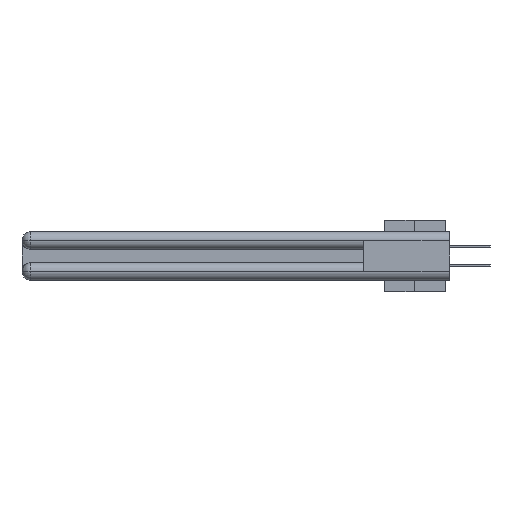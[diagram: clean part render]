
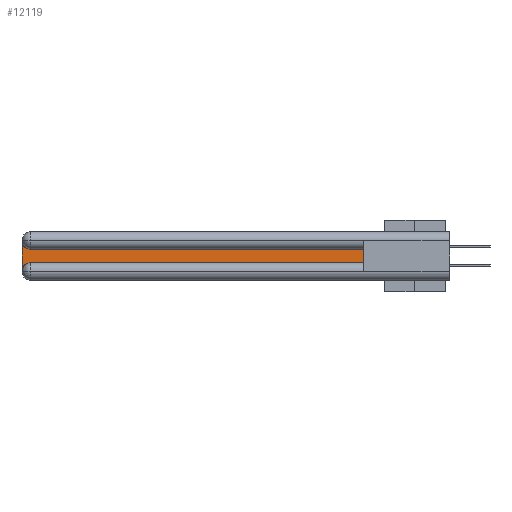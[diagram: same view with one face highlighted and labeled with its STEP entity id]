
A CAD part, left-side view. The second image highlights one B-rep face of the part: STEP entity #12119.
In plain terms, the highlighted planar face has unit normal (-1, 0, 0).
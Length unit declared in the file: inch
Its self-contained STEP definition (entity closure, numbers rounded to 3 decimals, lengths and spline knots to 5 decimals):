
#424 = AXIS2_PLACEMENT_3D ( 'NONE', #31968, #34974, #2307 ) ;
#792 = EDGE_CURVE ( 'NONE', #24513, #30034, #34742, .T. ) ;
#1741 = ORIENTED_EDGE ( 'NONE', *, *, #31828, .T. ) ;
#2096 = CIRCLE ( 'NONE', #424, 0.06 ) ;
#2307 = DIRECTION ( 'NONE',  ( 0., 0., -1. ) ) ;
#2764 = DIRECTION ( 'NONE',  ( 0., 0., -1. ) ) ;
#3702 = CARTESIAN_POINT ( 'NONE',  ( 0.075, 0.6, -0.1225 ) ) ;
#4654 = ORIENTED_EDGE ( 'NONE', *, *, #12943, .T. ) ;
#6123 = VECTOR ( 'NONE', #26142, 39.37008 ) ;
#6742 = ORIENTED_EDGE ( 'NONE', *, *, #37867, .T. ) ;
#6860 = CARTESIAN_POINT ( 'NONE',  ( 0.075, 0.6, -0.2175 ) ) ;
#7799 = EDGE_CURVE ( 'NONE', #8086, #32859, #38044, .T. ) ;
#8086 = VERTEX_POINT ( 'NONE', #24693 ) ;
#8830 = LINE ( 'NONE', #37646, #34863 ) ;
#9027 = LINE ( 'NONE', #6860, #10901 ) ;
#10901 = VECTOR ( 'NONE', #24483, 39.37008 ) ;
#11229 = FACE_OUTER_BOUND ( 'NONE', #14668, .T. ) ;
#11356 = EDGE_CURVE ( 'NONE', #32859, #20998, #31253, .T. ) ;
#12003 = ORIENTED_EDGE ( 'NONE', *, *, #792, .T. ) ;
#12119 = ADVANCED_FACE ( 'NONE', ( #11229 ), #26613, .F. ) ;
#12943 = EDGE_CURVE ( 'NONE', #29046, #8086, #8830, .T. ) ;
#13380 = CARTESIAN_POINT ( 'NONE',  ( 0.075, 0.6, -0.1225 ) ) ;
#14668 = EDGE_LOOP ( 'NONE', ( #12003, #6742, #4654, #15709, #33791, #1741 ) ) ;
#15709 = ORIENTED_EDGE ( 'NONE', *, *, #7799, .T. ) ;
#16176 = CARTESIAN_POINT ( 'NONE',  ( 0.075, 0.6, -0.2175 ) ) ;
#17313 = CARTESIAN_POINT ( 'NONE',  ( 0.075, 0.6, -0.2175 ) ) ;
#17334 = DIRECTION ( 'NONE',  ( 1., 0., 0. ) ) ;
#19529 = AXIS2_PLACEMENT_3D ( 'NONE', #32120, #29493, #38328 ) ;
#20998 = VERTEX_POINT ( 'NONE', #16176 ) ;
#21916 = AXIS2_PLACEMENT_3D ( 'NONE', #35039, #17334, #2764 ) ;
#24109 = DIRECTION ( 'NONE',  ( 0., 1., 0. ) ) ;
#24483 = DIRECTION ( 'NONE',  ( 0., 0., 1. ) ) ;
#24513 = VERTEX_POINT ( 'NONE', #13380 ) ;
#24693 = CARTESIAN_POINT ( 'NONE',  ( 0.075, 3., -0.2775 ) ) ;
#25141 = CARTESIAN_POINT ( 'NONE',  ( 0.075, 3., -0.0625 ) ) ;
#25368 = CARTESIAN_POINT ( 'NONE',  ( 0.075, 2.94, -0.1225 ) ) ;
#26142 = DIRECTION ( 'NONE',  ( 0., -1., 0. ) ) ;
#26491 = CARTESIAN_POINT ( 'NONE',  ( 0.075, 2.94, -0.2175 ) ) ;
#26613 = PLANE ( 'NONE',  #19529 ) ;
#29046 = VERTEX_POINT ( 'NONE', #25141 ) ;
#29493 = DIRECTION ( 'NONE',  ( 1., 0., 0. ) ) ;
#30034 = VERTEX_POINT ( 'NONE', #25368 ) ;
#31253 = LINE ( 'NONE', #17313, #6123 ) ;
#31828 = EDGE_CURVE ( 'NONE', #20998, #24513, #9027, .T. ) ;
#31968 = CARTESIAN_POINT ( 'NONE',  ( 0.075, 2.94, -0.0625 ) ) ;
#32120 = CARTESIAN_POINT ( 'NONE',  ( 0.075, 3., -0.1225 ) ) ;
#32859 = VERTEX_POINT ( 'NONE', #26491 ) ;
#33791 = ORIENTED_EDGE ( 'NONE', *, *, #11356, .T. ) ;
#34143 = DIRECTION ( 'NONE',  ( 0., 0., -1. ) ) ;
#34742 = LINE ( 'NONE', #3702, #37044 ) ;
#34863 = VECTOR ( 'NONE', #34143, 39.37008 ) ;
#34974 = DIRECTION ( 'NONE',  ( 1., 0., 0. ) ) ;
#35039 = CARTESIAN_POINT ( 'NONE',  ( 0.075, 2.94, -0.2775 ) ) ;
#37044 = VECTOR ( 'NONE', #24109, 39.37008 ) ;
#37646 = CARTESIAN_POINT ( 'NONE',  ( 0.075, 3., -0.2175 ) ) ;
#37867 = EDGE_CURVE ( 'NONE', #30034, #29046, #2096, .T. ) ;
#38044 = CIRCLE ( 'NONE', #21916, 0.06 ) ;
#38328 = DIRECTION ( 'NONE',  ( 0., 0., -1. ) ) ;
